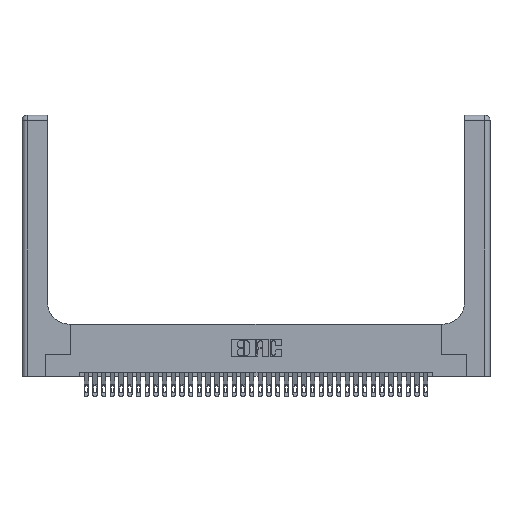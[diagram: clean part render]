
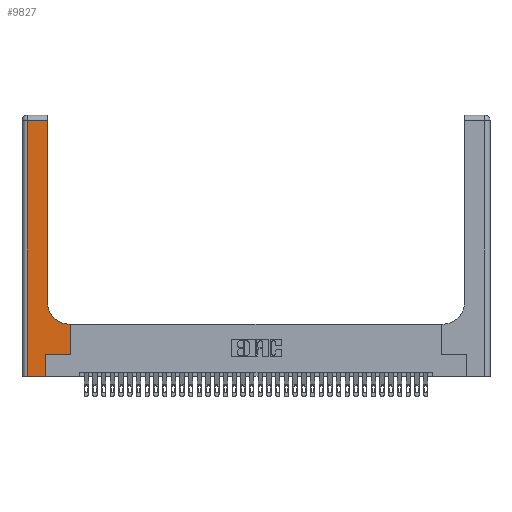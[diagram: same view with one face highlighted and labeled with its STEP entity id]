
A CAD part, top view. The second image highlights one B-rep face of the part: STEP entity #9827.
In plain terms, the highlighted planar face has unit normal (0, 0, 1).
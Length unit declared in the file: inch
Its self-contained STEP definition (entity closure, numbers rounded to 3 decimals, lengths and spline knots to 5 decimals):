
#150 = CARTESIAN_POINT ( 'NONE',  ( 0.5585, 0.25, 0.37 ) ) ;
#475 = ORIENTED_EDGE ( 'NONE', *, *, #28850, .T. ) ;
#761 = VERTEX_POINT ( 'NONE', #5388 ) ;
#925 = VECTOR ( 'NONE', #28126, 39.37008 ) ;
#1327 = VECTOR ( 'NONE', #26675, 39.37008 ) ;
#1394 = ORIENTED_EDGE ( 'NONE', *, *, #23035, .T. ) ;
#1421 = EDGE_CURVE ( 'NONE', #29793, #35633, #14806, .T. ) ;
#1953 = DIRECTION ( 'NONE',  ( 0., 1., 0. ) ) ;
#2245 = VECTOR ( 'NONE', #1953, 39.37008 ) ;
#2440 = CARTESIAN_POINT ( 'NONE',  ( 0.2915, 0.85, 0.37 ) ) ;
#2857 = LINE ( 'NONE', #7697, #24917 ) ;
#2899 = EDGE_LOOP ( 'NONE', ( #29731, #7710, #17207, #24807, #19888, #29295, #14965, #475, #1394 ) ) ;
#3611 = VECTOR ( 'NONE', #31034, 39.37008 ) ;
#4056 = LINE ( 'NONE', #7627, #2245 ) ;
#4391 = CARTESIAN_POINT ( 'NONE',  ( 0.06, 3., 0.37 ) ) ;
#4752 = VERTEX_POINT ( 'NONE', #8802 ) ;
#5060 = VERTEX_POINT ( 'NONE', #11696 ) ;
#5388 = CARTESIAN_POINT ( 'NONE',  ( 0.2915, 2.94, 0.37 ) ) ;
#6473 = VECTOR ( 'NONE', #33129, 39.37008 ) ;
#6488 = CARTESIAN_POINT ( 'NONE',  ( 0.5415, 0.85, 0.37 ) ) ;
#6599 = CIRCLE ( 'NONE', #12911, 0.25 ) ;
#6782 = VECTOR ( 'NONE', #11158, 39.37008 ) ;
#7627 = CARTESIAN_POINT ( 'NONE',  ( 0.2915, 3., 0.37 ) ) ;
#7697 = CARTESIAN_POINT ( 'NONE',  ( 0.269, 0.25, 0.37 ) ) ;
#7710 = ORIENTED_EDGE ( 'NONE', *, *, #28585, .T. ) ;
#8802 = CARTESIAN_POINT ( 'NONE',  ( 0.06, 0., 0.37 ) ) ;
#9384 = DIRECTION ( 'NONE',  ( 1., 0., 0. ) ) ;
#9827 = ADVANCED_FACE ( 'NONE', ( #29008 ), #11862, .F. ) ;
#10615 = DIRECTION ( 'NONE',  ( 1., 0., 0. ) ) ;
#10984 = CARTESIAN_POINT ( 'NONE',  ( 0.2915, 0.6, 0.37 ) ) ;
#11158 = DIRECTION ( 'NONE',  ( 0., 1., 0. ) ) ;
#11696 = CARTESIAN_POINT ( 'NONE',  ( 0.06, 2.94, 0.37 ) ) ;
#11862 = PLANE ( 'NONE',  #33080 ) ;
#12020 = VERTEX_POINT ( 'NONE', #2440 ) ;
#12905 = VECTOR ( 'NONE', #31837, 39.37008 ) ;
#12911 = AXIS2_PLACEMENT_3D ( 'NONE', #6488, #26573, #9384 ) ;
#14233 = EDGE_CURVE ( 'NONE', #12020, #761, #4056, .T. ) ;
#14756 = DIRECTION ( 'NONE',  ( 0., 0., -1. ) ) ;
#14806 = LINE ( 'NONE', #28313, #6782 ) ;
#14965 = ORIENTED_EDGE ( 'NONE', *, *, #1421, .T. ) ;
#14987 = VERTEX_POINT ( 'NONE', #28292 ) ;
#17207 = ORIENTED_EDGE ( 'NONE', *, *, #35285, .T. ) ;
#18180 = CARTESIAN_POINT ( 'NONE',  ( 0., 2.94, 0.37 ) ) ;
#19888 = ORIENTED_EDGE ( 'NONE', *, *, #24815, .T. ) ;
#20277 = CARTESIAN_POINT ( 'NONE',  ( 0.5585, 0.6, 0.37 ) ) ;
#23035 = EDGE_CURVE ( 'NONE', #30812, #12020, #6599, .T. ) ;
#23904 = LINE ( 'NONE', #31014, #925 ) ;
#24498 = VERTEX_POINT ( 'NONE', #30369 ) ;
#24807 = ORIENTED_EDGE ( 'NONE', *, *, #31961, .T. ) ;
#24815 = EDGE_CURVE ( 'NONE', #24498, #14987, #28140, .T. ) ;
#24917 = VECTOR ( 'NONE', #10615, 39.37008 ) ;
#26148 = CARTESIAN_POINT ( 'NONE',  ( 0., 3., 0.37 ) ) ;
#26573 = DIRECTION ( 'NONE',  ( 0., 0., -1. ) ) ;
#26675 = DIRECTION ( 'NONE',  ( -1., 0., 0. ) ) ;
#28126 = DIRECTION ( 'NONE',  ( 1., 0., 0. ) ) ;
#28140 = LINE ( 'NONE', #28964, #12905 ) ;
#28292 = CARTESIAN_POINT ( 'NONE',  ( 0.269, 0.25, 0.37 ) ) ;
#28313 = CARTESIAN_POINT ( 'NONE',  ( 0.5585, 0.25, 0.37 ) ) ;
#28585 = EDGE_CURVE ( 'NONE', #761, #5060, #31907, .T. ) ;
#28770 = CARTESIAN_POINT ( 'NONE',  ( 0.5415, 0.6, 0.37 ) ) ;
#28850 = EDGE_CURVE ( 'NONE', #35633, #30812, #31452, .T. ) ;
#28964 = CARTESIAN_POINT ( 'NONE',  ( 0.269, 0., 0.37 ) ) ;
#29008 = FACE_OUTER_BOUND ( 'NONE', #2899, .T. ) ;
#29295 = ORIENTED_EDGE ( 'NONE', *, *, #30574, .T. ) ;
#29731 = ORIENTED_EDGE ( 'NONE', *, *, #14233, .T. ) ;
#29793 = VERTEX_POINT ( 'NONE', #150 ) ;
#30281 = LINE ( 'NONE', #4391, #6473 ) ;
#30369 = CARTESIAN_POINT ( 'NONE',  ( 0.269, 0., 0.37 ) ) ;
#30574 = EDGE_CURVE ( 'NONE', #14987, #29793, #2857, .T. ) ;
#30812 = VERTEX_POINT ( 'NONE', #28770 ) ;
#31014 = CARTESIAN_POINT ( 'NONE',  ( 0., 0., 0.37 ) ) ;
#31034 = DIRECTION ( 'NONE',  ( -1., 0., 0. ) ) ;
#31452 = LINE ( 'NONE', #10984, #3611 ) ;
#31837 = DIRECTION ( 'NONE',  ( 0., 1., 0. ) ) ;
#31907 = LINE ( 'NONE', #18180, #1327 ) ;
#31961 = EDGE_CURVE ( 'NONE', #4752, #24498, #23904, .T. ) ;
#33080 = AXIS2_PLACEMENT_3D ( 'NONE', #26148, #14756, #34763 ) ;
#33129 = DIRECTION ( 'NONE',  ( 0., -1., 0. ) ) ;
#34763 = DIRECTION ( 'NONE',  ( -1., 0., 0. ) ) ;
#35285 = EDGE_CURVE ( 'NONE', #5060, #4752, #30281, .T. ) ;
#35633 = VERTEX_POINT ( 'NONE', #20277 ) ;
